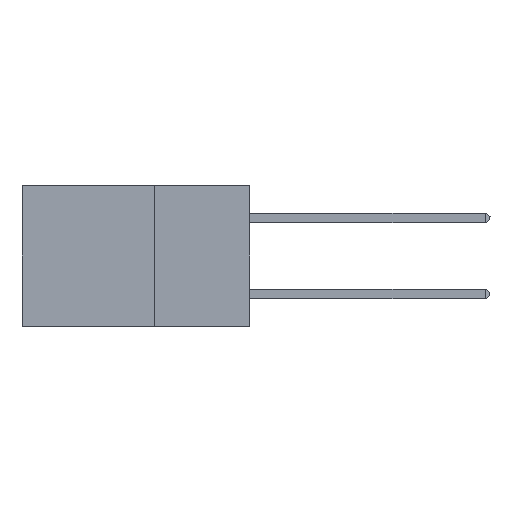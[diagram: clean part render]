
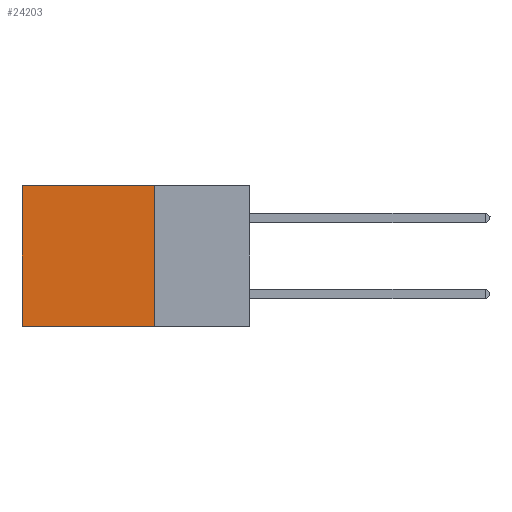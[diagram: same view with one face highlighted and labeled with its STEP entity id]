
A CAD part, left-side view. The second image highlights one B-rep face of the part: STEP entity #24203.
In plain terms, the highlighted planar face has unit normal (-1, 0, 0).
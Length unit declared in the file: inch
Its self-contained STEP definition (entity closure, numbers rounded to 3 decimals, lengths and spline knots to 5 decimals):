
#2075 = PLANE ( 'NONE',  #36856 ) ;
#5325 = ORIENTED_EDGE ( 'NONE', *, *, #36350, .T. ) ;
#8587 = EDGE_CURVE ( 'NONE', #10369, #17931, #28087, .T. ) ;
#10275 = DIRECTION ( 'NONE',  ( 0., 1., 0. ) ) ;
#10324 = VERTEX_POINT ( 'NONE', #37339 ) ;
#10369 = VERTEX_POINT ( 'NONE', #21934 ) ;
#11090 = FACE_OUTER_BOUND ( 'NONE', #32470, .T. ) ;
#11420 = ORIENTED_EDGE ( 'NONE', *, *, #31087, .F. ) ;
#12917 = ORIENTED_EDGE ( 'NONE', *, *, #8587, .F. ) ;
#12947 = ORIENTED_EDGE ( 'NONE', *, *, #19027, .T. ) ;
#14584 = DIRECTION ( 'NONE',  ( 1., 0., 0. ) ) ;
#15043 = VECTOR ( 'NONE', #10275, 39.37008 ) ;
#15640 = LINE ( 'NONE', #31258, #35639 ) ;
#15755 = DIRECTION ( 'NONE',  ( 0., 0., -1. ) ) ;
#16193 = CARTESIAN_POINT ( 'NONE',  ( 0.2875, 0.6, 0. ) ) ;
#17931 = VERTEX_POINT ( 'NONE', #24188 ) ;
#19027 = EDGE_CURVE ( 'NONE', #10369, #32581, #37994, .T. ) ;
#19682 = CARTESIAN_POINT ( 'NONE',  ( 0.2875, 0.25, -0.37 ) ) ;
#19880 = LINE ( 'NONE', #19682, #40448 ) ;
#21934 = CARTESIAN_POINT ( 'NONE',  ( 0.2875, 0.25, 0. ) ) ;
#24188 = CARTESIAN_POINT ( 'NONE',  ( 0.2875, 0.25, -0.37 ) ) ;
#24203 = ADVANCED_FACE ( 'NONE', ( #11090 ), #2075, .F. ) ;
#25621 = CARTESIAN_POINT ( 'NONE',  ( 0.2875, 0.25, 0. ) ) ;
#27100 = CARTESIAN_POINT ( 'NONE',  ( 0.2875, 0.25, 0. ) ) ;
#27215 = DIRECTION ( 'NONE',  ( 0., 0., -1. ) ) ;
#28087 = LINE ( 'NONE', #25621, #36697 ) ;
#28720 = DIRECTION ( 'NONE',  ( 0., 1., 0. ) ) ;
#31087 = EDGE_CURVE ( 'NONE', #17931, #10324, #19880, .T. ) ;
#31258 = CARTESIAN_POINT ( 'NONE',  ( 0.2875, 0.6, 0. ) ) ;
#32470 = EDGE_LOOP ( 'NONE', ( #5325, #11420, #12917, #12947 ) ) ;
#32581 = VERTEX_POINT ( 'NONE', #16193 ) ;
#33476 = DIRECTION ( 'NONE',  ( 0., 0., -1. ) ) ;
#35639 = VECTOR ( 'NONE', #27215, 39.37008 ) ;
#36350 = EDGE_CURVE ( 'NONE', #32581, #10324, #15640, .T. ) ;
#36697 = VECTOR ( 'NONE', #15755, 39.37008 ) ;
#36856 = AXIS2_PLACEMENT_3D ( 'NONE', #27100, #14584, #33476 ) ;
#37339 = CARTESIAN_POINT ( 'NONE',  ( 0.2875, 0.6, -0.37 ) ) ;
#37994 = LINE ( 'NONE', #38421, #15043 ) ;
#38421 = CARTESIAN_POINT ( 'NONE',  ( 0.2875, 0.25, 0. ) ) ;
#40448 = VECTOR ( 'NONE', #28720, 39.37008 ) ;
